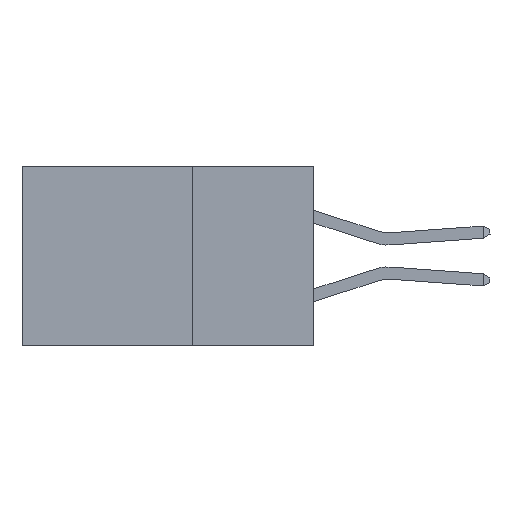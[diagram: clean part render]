
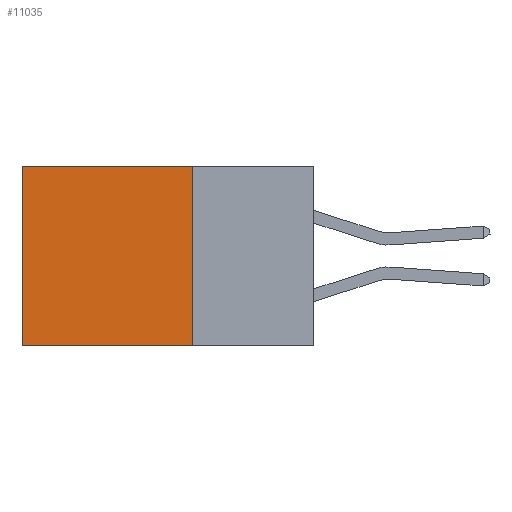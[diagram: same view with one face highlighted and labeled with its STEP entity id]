
A CAD part, left-side view. The second image highlights one B-rep face of the part: STEP entity #11035.
In plain terms, the highlighted planar face has unit normal (-1, 0, 0).
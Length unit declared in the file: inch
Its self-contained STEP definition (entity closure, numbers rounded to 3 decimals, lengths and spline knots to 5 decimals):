
#1089 = VERTEX_POINT ( 'NONE', #5868 ) ;
#1375 = LINE ( 'NONE', #28477, #29748 ) ;
#3616 = DIRECTION ( 'NONE',  ( 0., 1., 0. ) ) ;
#3808 = DIRECTION ( 'NONE',  ( 0., 0., -1. ) ) ;
#4161 = LINE ( 'NONE', #31482, #40777 ) ;
#5868 = CARTESIAN_POINT ( 'NONE',  ( 0.2875, 0.25, -0.37 ) ) ;
#6743 = ORIENTED_EDGE ( 'NONE', *, *, #42491, .F. ) ;
#7371 = VERTEX_POINT ( 'NONE', #22037 ) ;
#7487 = LINE ( 'NONE', #24247, #31336 ) ;
#7809 = ORIENTED_EDGE ( 'NONE', *, *, #23714, .T. ) ;
#8633 = DIRECTION ( 'NONE',  ( 0., 0., -1. ) ) ;
#10054 = VECTOR ( 'NONE', #8633, 39.37008 ) ;
#10655 = CARTESIAN_POINT ( 'NONE',  ( 0.2875, 0.6, 0. ) ) ;
#11035 = ADVANCED_FACE ( 'NONE', ( #32148 ), #42562, .F. ) ;
#13318 = VERTEX_POINT ( 'NONE', #10655 ) ;
#21518 = CARTESIAN_POINT ( 'NONE',  ( 0.2875, 0.25, 0. ) ) ;
#22037 = CARTESIAN_POINT ( 'NONE',  ( 0.2875, 0.6, -0.37 ) ) ;
#22180 = EDGE_LOOP ( 'NONE', ( #34859, #36171, #6743, #7809 ) ) ;
#23714 = EDGE_CURVE ( 'NONE', #30835, #13318, #1375, .T. ) ;
#24247 = CARTESIAN_POINT ( 'NONE',  ( 0.2875, 0.25, -0.37 ) ) ;
#24311 = EDGE_CURVE ( 'NONE', #1089, #7371, #7487, .T. ) ;
#25101 = DIRECTION ( 'NONE',  ( 1., 0., 0. ) ) ;
#26719 = CARTESIAN_POINT ( 'NONE',  ( 0.2875, 0.25, 0. ) ) ;
#28477 = CARTESIAN_POINT ( 'NONE',  ( 0.2875, 0.25, 0. ) ) ;
#29070 = EDGE_CURVE ( 'NONE', #13318, #7371, #4161, .T. ) ;
#29748 = VECTOR ( 'NONE', #3616, 39.37008 ) ;
#30031 = LINE ( 'NONE', #36988, #10054 ) ;
#30835 = VERTEX_POINT ( 'NONE', #26719 ) ;
#31336 = VECTOR ( 'NONE', #35066, 39.37008 ) ;
#31482 = CARTESIAN_POINT ( 'NONE',  ( 0.2875, 0.6, 0. ) ) ;
#32148 = FACE_OUTER_BOUND ( 'NONE', #22180, .T. ) ;
#34859 = ORIENTED_EDGE ( 'NONE', *, *, #29070, .T. ) ;
#35066 = DIRECTION ( 'NONE',  ( 0., 1., 0. ) ) ;
#35205 = DIRECTION ( 'NONE',  ( 0., 0., -1. ) ) ;
#35779 = AXIS2_PLACEMENT_3D ( 'NONE', #21518, #25101, #3808 ) ;
#36171 = ORIENTED_EDGE ( 'NONE', *, *, #24311, .F. ) ;
#36988 = CARTESIAN_POINT ( 'NONE',  ( 0.2875, 0.25, 0. ) ) ;
#40777 = VECTOR ( 'NONE', #35205, 39.37008 ) ;
#42491 = EDGE_CURVE ( 'NONE', #30835, #1089, #30031, .T. ) ;
#42562 = PLANE ( 'NONE',  #35779 ) ;
